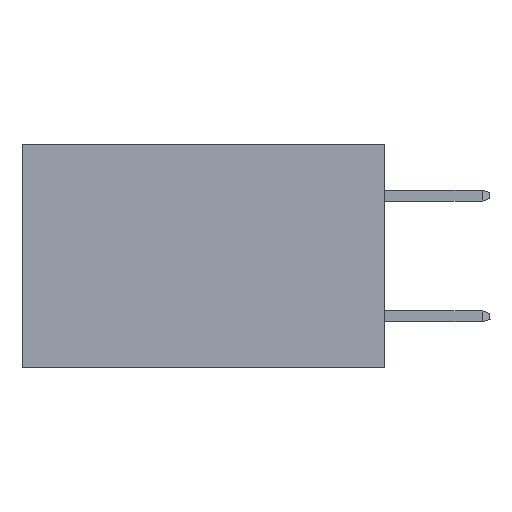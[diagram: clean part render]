
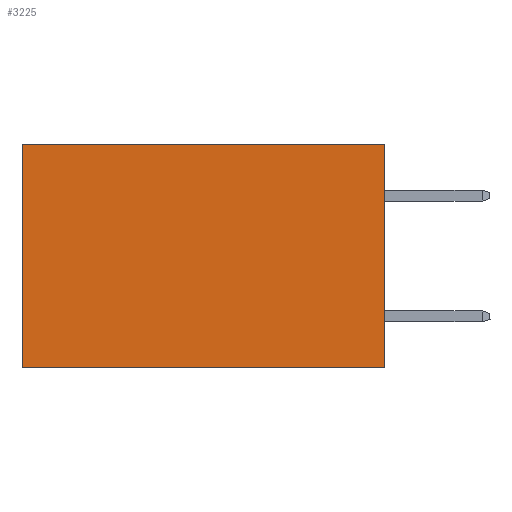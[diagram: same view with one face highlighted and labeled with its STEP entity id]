
A CAD part, left-side view. The second image highlights one B-rep face of the part: STEP entity #3225.
In plain terms, the highlighted planar face has unit normal (-1, 0, 0).
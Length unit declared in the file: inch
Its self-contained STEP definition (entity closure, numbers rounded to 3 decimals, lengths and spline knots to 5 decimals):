
#41 = DIRECTION ( 'NONE',  ( 0., 0., -1. ) ) ;
#262 = AXIS2_PLACEMENT_3D ( 'NONE', #11621, #12248, #12217 ) ;
#1077 = LINE ( 'NONE', #23163, #5507 ) ;
#1719 = CARTESIAN_POINT ( 'NONE',  ( 0.2615, 0.6, -0.37 ) ) ;
#2034 = VERTEX_POINT ( 'NONE', #11516 ) ;
#3092 = LINE ( 'NONE', #23789, #17617 ) ;
#3225 = ADVANCED_FACE ( 'NONE', ( #23110 ), #11915, .F. ) ;
#3428 = EDGE_CURVE ( 'NONE', #2034, #15480, #23395, .T. ) ;
#3585 = EDGE_CURVE ( 'NONE', #24246, #2034, #1077, .T. ) ;
#4781 = DIRECTION ( 'NONE',  ( 0., 0., -1. ) ) ;
#5507 = VECTOR ( 'NONE', #41, 39.37008 ) ;
#6845 = VECTOR ( 'NONE', #4781, 39.37008 ) ;
#6931 = ORIENTED_EDGE ( 'NONE', *, *, #3428, .F. ) ;
#9304 = DIRECTION ( 'NONE',  ( 0., 1., 0. ) ) ;
#10064 = CARTESIAN_POINT ( 'NONE',  ( 0.2615, 0., 0. ) ) ;
#10425 = CARTESIAN_POINT ( 'NONE',  ( 0.2615, 0., -0.37 ) ) ;
#11516 = CARTESIAN_POINT ( 'NONE',  ( 0.2615, 0., -0.37 ) ) ;
#11621 = CARTESIAN_POINT ( 'NONE',  ( 0.2615, 0., -0.37 ) ) ;
#11864 = VERTEX_POINT ( 'NONE', #21467 ) ;
#11915 = PLANE ( 'NONE',  #262 ) ;
#11971 = LINE ( 'NONE', #23463, #6845 ) ;
#12217 = DIRECTION ( 'NONE',  ( 0., 0., -1. ) ) ;
#12248 = DIRECTION ( 'NONE',  ( 1., 0., 0. ) ) ;
#13357 = ORIENTED_EDGE ( 'NONE', *, *, #3585, .F. ) ;
#13756 = EDGE_LOOP ( 'NONE', ( #22024, #6931, #13357, #16618 ) ) ;
#14577 = DIRECTION ( 'NONE',  ( 0., 1., 0. ) ) ;
#15480 = VERTEX_POINT ( 'NONE', #1719 ) ;
#16618 = ORIENTED_EDGE ( 'NONE', *, *, #17984, .T. ) ;
#17617 = VECTOR ( 'NONE', #14577, 39.37008 ) ;
#17984 = EDGE_CURVE ( 'NONE', #24246, #11864, #3092, .T. ) ;
#18507 = VECTOR ( 'NONE', #9304, 39.37008 ) ;
#20291 = EDGE_CURVE ( 'NONE', #11864, #15480, #11971, .T. ) ;
#21467 = CARTESIAN_POINT ( 'NONE',  ( 0.2615, 0.6, 0. ) ) ;
#22024 = ORIENTED_EDGE ( 'NONE', *, *, #20291, .T. ) ;
#23110 = FACE_OUTER_BOUND ( 'NONE', #13756, .T. ) ;
#23163 = CARTESIAN_POINT ( 'NONE',  ( 0.2615, 0., -0.37 ) ) ;
#23395 = LINE ( 'NONE', #10425, #18507 ) ;
#23463 = CARTESIAN_POINT ( 'NONE',  ( 0.2615, 0.6, -0.37 ) ) ;
#23789 = CARTESIAN_POINT ( 'NONE',  ( 0.2615, 0., 0. ) ) ;
#24246 = VERTEX_POINT ( 'NONE', #10064 ) ;
